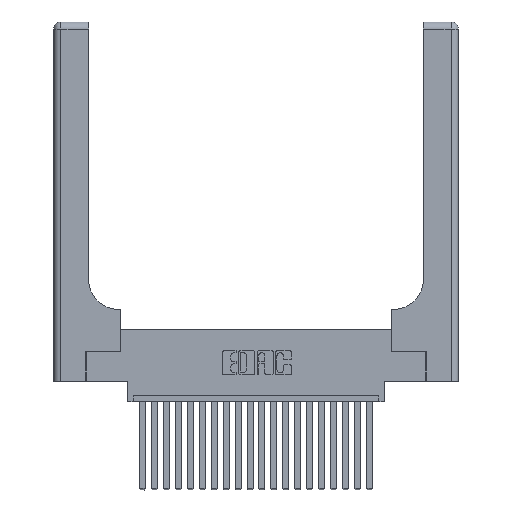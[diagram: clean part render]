
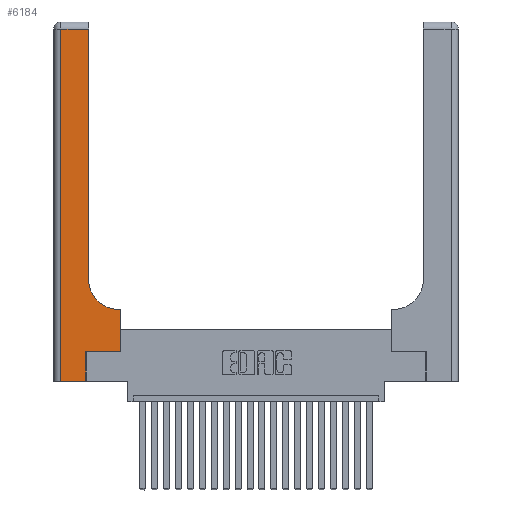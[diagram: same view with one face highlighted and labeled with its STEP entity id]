
A CAD part, top view. The second image highlights one B-rep face of the part: STEP entity #6184.
In plain terms, the highlighted planar face has unit normal (0, 0, 1).
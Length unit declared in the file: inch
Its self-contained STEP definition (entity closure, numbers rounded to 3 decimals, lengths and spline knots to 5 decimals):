
#78 = CARTESIAN_POINT ( 'NONE',  ( 0., 0., 0.37 ) ) ;
#173 = EDGE_CURVE ( 'NONE', #9159, #1871, #9259, .T. ) ;
#276 = ORIENTED_EDGE ( 'NONE', *, *, #3567, .T. ) ;
#604 = DIRECTION ( 'NONE',  ( -1., 0., 0. ) ) ;
#705 = ORIENTED_EDGE ( 'NONE', *, *, #1147, .T. ) ;
#808 = FACE_OUTER_BOUND ( 'NONE', #9441, .T. ) ;
#1147 = EDGE_CURVE ( 'NONE', #13231, #5392, #8667, .T. ) ;
#1871 = VERTEX_POINT ( 'NONE', #22870 ) ;
#2576 = VERTEX_POINT ( 'NONE', #17372 ) ;
#2585 = DIRECTION ( 'NONE',  ( 0., 0., -1. ) ) ;
#2732 = ORIENTED_EDGE ( 'NONE', *, *, #173, .T. ) ;
#3567 = EDGE_CURVE ( 'NONE', #1871, #20047, #15770, .T. ) ;
#3581 = ORIENTED_EDGE ( 'NONE', *, *, #22060, .T. ) ;
#3865 = CARTESIAN_POINT ( 'NONE',  ( 0.2915, 0.6, 0.37 ) ) ;
#3945 = DIRECTION ( 'NONE',  ( -1., 0., 0. ) ) ;
#4064 = EDGE_CURVE ( 'NONE', #6488, #11343, #21659, .T. ) ;
#4316 = VECTOR ( 'NONE', #604, 39.37008 ) ;
#4357 = CARTESIAN_POINT ( 'NONE',  ( 0.5585, 0.25, 0.37 ) ) ;
#4488 = CARTESIAN_POINT ( 'NONE',  ( 0.2915, 0.85, 0.37 ) ) ;
#4538 = VECTOR ( 'NONE', #5812, 39.37008 ) ;
#5290 = EDGE_CURVE ( 'NONE', #8474, #9159, #16547, .T. ) ;
#5392 = VERTEX_POINT ( 'NONE', #22754 ) ;
#5784 = PLANE ( 'NONE',  #7964 ) ;
#5812 = DIRECTION ( 'NONE',  ( 1., 0., 0. ) ) ;
#6184 = ADVANCED_FACE ( 'NONE', ( #808 ), #5784, .F. ) ;
#6263 = LINE ( 'NONE', #17164, #18024 ) ;
#6488 = VERTEX_POINT ( 'NONE', #15997 ) ;
#6883 = CARTESIAN_POINT ( 'NONE',  ( 0.269, 0., 0.37 ) ) ;
#6897 = AXIS2_PLACEMENT_3D ( 'NONE', #21929, #11209, #9496 ) ;
#7964 = AXIS2_PLACEMENT_3D ( 'NONE', #10089, #2585, #13569 ) ;
#8474 = VERTEX_POINT ( 'NONE', #10208 ) ;
#8667 = LINE ( 'NONE', #12520, #17885 ) ;
#8786 = DIRECTION ( 'NONE',  ( 0., 1., 0. ) ) ;
#9079 = VECTOR ( 'NONE', #22902, 39.37008 ) ;
#9080 = EDGE_CURVE ( 'NONE', #11343, #2576, #6263, .T. ) ;
#9159 = VERTEX_POINT ( 'NONE', #4488 ) ;
#9259 = LINE ( 'NONE', #17600, #19596 ) ;
#9279 = ORIENTED_EDGE ( 'NONE', *, *, #5290, .T. ) ;
#9441 = EDGE_LOOP ( 'NONE', ( #2732, #276, #3581, #18110, #9833, #11158, #705, #19931, #9279 ) ) ;
#9496 = DIRECTION ( 'NONE',  ( 1., 0., 0. ) ) ;
#9833 = ORIENTED_EDGE ( 'NONE', *, *, #9080, .T. ) ;
#10089 = CARTESIAN_POINT ( 'NONE',  ( 0., 3., 0.37 ) ) ;
#10208 = CARTESIAN_POINT ( 'NONE',  ( 0.5415, 0.6, 0.37 ) ) ;
#11158 = ORIENTED_EDGE ( 'NONE', *, *, #15181, .T. ) ;
#11209 = DIRECTION ( 'NONE',  ( 0., 0., -1. ) ) ;
#11343 = VERTEX_POINT ( 'NONE', #6883 ) ;
#11763 = CARTESIAN_POINT ( 'NONE',  ( 0., 2.94, 0.37 ) ) ;
#12369 = DIRECTION ( 'NONE',  ( 0., 1., 0. ) ) ;
#12520 = CARTESIAN_POINT ( 'NONE',  ( 0.5585, 0.25, 0.37 ) ) ;
#13231 = VERTEX_POINT ( 'NONE', #4357 ) ;
#13569 = DIRECTION ( 'NONE',  ( -1., 0., 0. ) ) ;
#13794 = LINE ( 'NONE', #15681, #9079 ) ;
#15181 = EDGE_CURVE ( 'NONE', #2576, #13231, #22196, .T. ) ;
#15681 = CARTESIAN_POINT ( 'NONE',  ( 0.06, 3., 0.37 ) ) ;
#15770 = LINE ( 'NONE', #11763, #4316 ) ;
#15997 = CARTESIAN_POINT ( 'NONE',  ( 0.06, 0., 0.37 ) ) ;
#16547 = CIRCLE ( 'NONE', #6897, 0.25 ) ;
#17136 = VECTOR ( 'NONE', #3945, 39.37008 ) ;
#17164 = CARTESIAN_POINT ( 'NONE',  ( 0.269, 0., 0.37 ) ) ;
#17372 = CARTESIAN_POINT ( 'NONE',  ( 0.269, 0.25, 0.37 ) ) ;
#17405 = DIRECTION ( 'NONE',  ( 0., 1., 0. ) ) ;
#17600 = CARTESIAN_POINT ( 'NONE',  ( 0.2915, 3., 0.37 ) ) ;
#17885 = VECTOR ( 'NONE', #12369, 39.37008 ) ;
#18024 = VECTOR ( 'NONE', #17405, 39.37008 ) ;
#18110 = ORIENTED_EDGE ( 'NONE', *, *, #4064, .T. ) ;
#19596 = VECTOR ( 'NONE', #8786, 39.37008 ) ;
#19931 = ORIENTED_EDGE ( 'NONE', *, *, #22263, .T. ) ;
#20047 = VERTEX_POINT ( 'NONE', #20859 ) ;
#20242 = LINE ( 'NONE', #3865, #17136 ) ;
#20304 = DIRECTION ( 'NONE',  ( 1., 0., 0. ) ) ;
#20807 = VECTOR ( 'NONE', #20304, 39.37008 ) ;
#20859 = CARTESIAN_POINT ( 'NONE',  ( 0.06, 2.94, 0.37 ) ) ;
#21410 = CARTESIAN_POINT ( 'NONE',  ( 0.269, 0.25, 0.37 ) ) ;
#21659 = LINE ( 'NONE', #78, #20807 ) ;
#21929 = CARTESIAN_POINT ( 'NONE',  ( 0.5415, 0.85, 0.37 ) ) ;
#22060 = EDGE_CURVE ( 'NONE', #20047, #6488, #13794, .T. ) ;
#22196 = LINE ( 'NONE', #21410, #4538 ) ;
#22263 = EDGE_CURVE ( 'NONE', #5392, #8474, #20242, .T. ) ;
#22754 = CARTESIAN_POINT ( 'NONE',  ( 0.5585, 0.6, 0.37 ) ) ;
#22870 = CARTESIAN_POINT ( 'NONE',  ( 0.2915, 2.94, 0.37 ) ) ;
#22902 = DIRECTION ( 'NONE',  ( 0., -1., 0. ) ) ;
